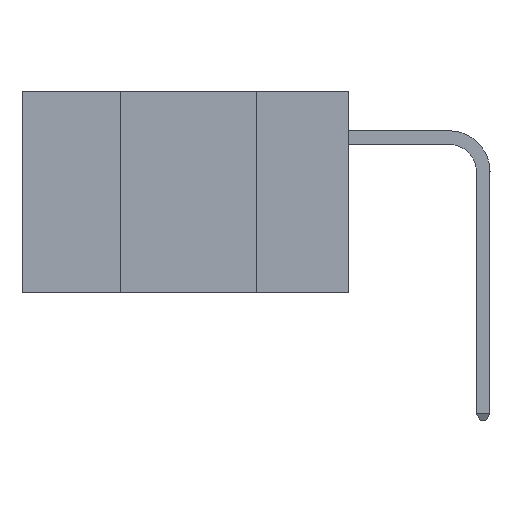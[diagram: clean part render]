
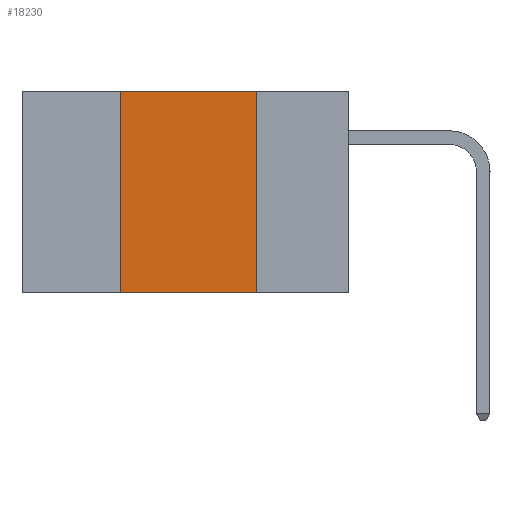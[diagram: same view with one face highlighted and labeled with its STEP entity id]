
A CAD part, left-side view. The second image highlights one B-rep face of the part: STEP entity #18230.
In plain terms, the highlighted planar face has unit normal (-1, 0, 0).
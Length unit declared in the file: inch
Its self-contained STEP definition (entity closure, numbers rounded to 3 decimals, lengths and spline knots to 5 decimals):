
#176 = CARTESIAN_POINT ( 'NONE',  ( 0., 0.42, 0. ) ) ;
#326 = DIRECTION ( 'NONE',  ( 0., -1., 0. ) ) ;
#913 = DIRECTION ( 'NONE',  ( 0., -1., 0. ) ) ;
#1172 = ORIENTED_EDGE ( 'NONE', *, *, #8101, .T. ) ;
#1555 = CARTESIAN_POINT ( 'NONE',  ( 0., 0.17, 0. ) ) ;
#2046 = VERTEX_POINT ( 'NONE', #4127 ) ;
#2257 = EDGE_CURVE ( 'NONE', #4641, #8385, #14108, .T. ) ;
#3269 = ORIENTED_EDGE ( 'NONE', *, *, #2257, .F. ) ;
#3457 = DIRECTION ( 'NONE',  ( 0., 0., 1. ) ) ;
#3867 = ORIENTED_EDGE ( 'NONE', *, *, #9572, .F. ) ;
#3986 = LINE ( 'NONE', #1555, #10539 ) ;
#4127 = CARTESIAN_POINT ( 'NONE',  ( 0., 0.17, -0.37 ) ) ;
#4641 = VERTEX_POINT ( 'NONE', #176 ) ;
#4705 = ORIENTED_EDGE ( 'NONE', *, *, #15457, .F. ) ;
#4948 = VECTOR ( 'NONE', #326, 39.37008 ) ;
#4966 = CARTESIAN_POINT ( 'NONE',  ( 0., 0.42, 0. ) ) ;
#6175 = AXIS2_PLACEMENT_3D ( 'NONE', #13263, #14685, #6456 ) ;
#6456 = DIRECTION ( 'NONE',  ( 0., 0., -1. ) ) ;
#6866 = CARTESIAN_POINT ( 'NONE',  ( 0., 0.6, 0. ) ) ;
#8101 = EDGE_CURVE ( 'NONE', #15742, #2046, #15944, .T. ) ;
#8385 = VERTEX_POINT ( 'NONE', #12444 ) ;
#9572 = EDGE_CURVE ( 'NONE', #8385, #2046, #3986, .T. ) ;
#10371 = CARTESIAN_POINT ( 'NONE',  ( 0., 0.6, -0.37 ) ) ;
#10400 = VECTOR ( 'NONE', #913, 39.37008 ) ;
#10539 = VECTOR ( 'NONE', #15587, 39.37008 ) ;
#12444 = CARTESIAN_POINT ( 'NONE',  ( 0., 0.17, 0. ) ) ;
#12681 = FACE_OUTER_BOUND ( 'NONE', #13001, .T. ) ;
#13001 = EDGE_LOOP ( 'NONE', ( #3867, #3269, #4705, #1172 ) ) ;
#13195 = VECTOR ( 'NONE', #3457, 39.37008 ) ;
#13263 = CARTESIAN_POINT ( 'NONE',  ( 0., 0.6, 0. ) ) ;
#13324 = PLANE ( 'NONE',  #6175 ) ;
#13993 = CARTESIAN_POINT ( 'NONE',  ( 0., 0.42, -0.37 ) ) ;
#14108 = LINE ( 'NONE', #6866, #10400 ) ;
#14685 = DIRECTION ( 'NONE',  ( 1., 0., 0. ) ) ;
#15457 = EDGE_CURVE ( 'NONE', #15742, #4641, #16808, .T. ) ;
#15587 = DIRECTION ( 'NONE',  ( 0., 0., -1. ) ) ;
#15742 = VERTEX_POINT ( 'NONE', #13993 ) ;
#15944 = LINE ( 'NONE', #10371, #4948 ) ;
#16808 = LINE ( 'NONE', #4966, #13195 ) ;
#18230 = ADVANCED_FACE ( 'NONE', ( #12681 ), #13324, .F. ) ;
